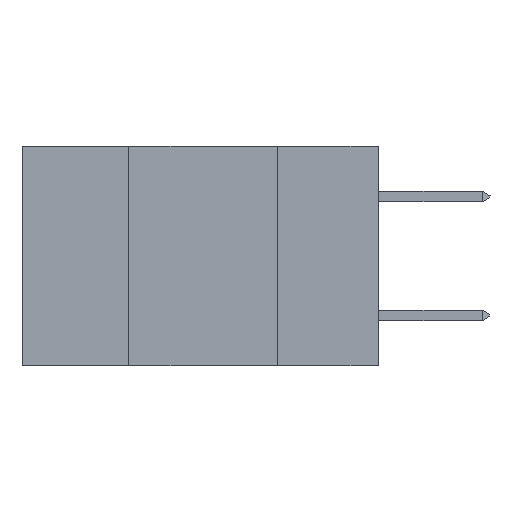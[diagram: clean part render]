
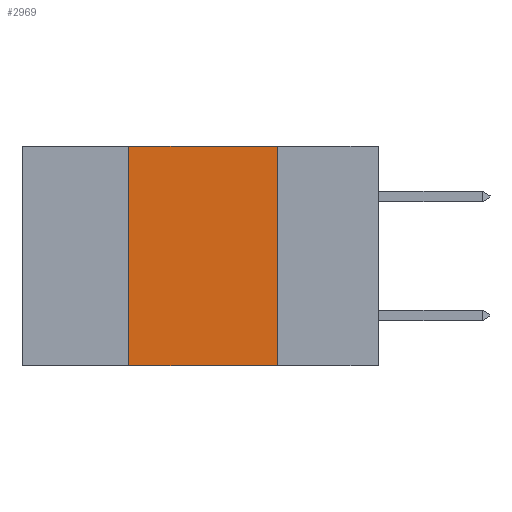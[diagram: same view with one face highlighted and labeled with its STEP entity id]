
A CAD part, left-side view. The second image highlights one B-rep face of the part: STEP entity #2969.
In plain terms, the highlighted planar face has unit normal (-1, 0, 0).
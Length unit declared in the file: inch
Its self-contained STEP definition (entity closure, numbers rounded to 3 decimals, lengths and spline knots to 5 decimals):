
#206 = AXIS2_PLACEMENT_3D ( 'NONE', #6685, #3873, #6590 ) ;
#290 = CARTESIAN_POINT ( 'NONE',  ( 0., 0.42, -0.37 ) ) ;
#675 = VECTOR ( 'NONE', #8273, 39.37008 ) ;
#930 = DIRECTION ( 'NONE',  ( 0., 0., -1. ) ) ;
#960 = VERTEX_POINT ( 'NONE', #290 ) ;
#1196 = PLANE ( 'NONE',  #206 ) ;
#1457 = LINE ( 'NONE', #4963, #675 ) ;
#1615 = CARTESIAN_POINT ( 'NONE',  ( 0., 0.17, 0. ) ) ;
#1866 = LINE ( 'NONE', #7361, #2971 ) ;
#1905 = EDGE_CURVE ( 'NONE', #960, #2613, #1866, .T. ) ;
#1963 = FACE_OUTER_BOUND ( 'NONE', #2246, .T. ) ;
#2007 = ORIENTED_EDGE ( 'NONE', *, *, #1905, .T. ) ;
#2048 = EDGE_CURVE ( 'NONE', #960, #8710, #7656, .T. ) ;
#2240 = ORIENTED_EDGE ( 'NONE', *, *, #2048, .F. ) ;
#2246 = EDGE_LOOP ( 'NONE', ( #3797, #7391, #2240, #2007 ) ) ;
#2274 = LINE ( 'NONE', #7089, #4988 ) ;
#2612 = DIRECTION ( 'NONE',  ( 0., -1., 0. ) ) ;
#2613 = VERTEX_POINT ( 'NONE', #2953 ) ;
#2637 = VERTEX_POINT ( 'NONE', #1615 ) ;
#2910 = DIRECTION ( 'NONE',  ( 0., 0., 1. ) ) ;
#2953 = CARTESIAN_POINT ( 'NONE',  ( 0., 0.17, -0.37 ) ) ;
#2969 = ADVANCED_FACE ( 'NONE', ( #1963 ), #1196, .F. ) ;
#2971 = VECTOR ( 'NONE', #2612, 39.37008 ) ;
#3797 = ORIENTED_EDGE ( 'NONE', *, *, #3976, .F. ) ;
#3873 = DIRECTION ( 'NONE',  ( 1., 0., 0. ) ) ;
#3976 = EDGE_CURVE ( 'NONE', #2637, #2613, #2274, .T. ) ;
#4720 = CARTESIAN_POINT ( 'NONE',  ( 0., 0.42, 0. ) ) ;
#4963 = CARTESIAN_POINT ( 'NONE',  ( 0., 0.6, 0. ) ) ;
#4988 = VECTOR ( 'NONE', #930, 39.37008 ) ;
#5397 = EDGE_CURVE ( 'NONE', #8710, #2637, #1457, .T. ) ;
#5407 = CARTESIAN_POINT ( 'NONE',  ( 0., 0.42, -0.37 ) ) ;
#6590 = DIRECTION ( 'NONE',  ( 0., 0., -1. ) ) ;
#6685 = CARTESIAN_POINT ( 'NONE',  ( 0., 0.6, 0. ) ) ;
#7089 = CARTESIAN_POINT ( 'NONE',  ( 0., 0.17, -0.37 ) ) ;
#7329 = VECTOR ( 'NONE', #2910, 39.37008 ) ;
#7361 = CARTESIAN_POINT ( 'NONE',  ( 0., 0.6, -0.37 ) ) ;
#7391 = ORIENTED_EDGE ( 'NONE', *, *, #5397, .F. ) ;
#7656 = LINE ( 'NONE', #5407, #7329 ) ;
#8273 = DIRECTION ( 'NONE',  ( 0., -1., 0. ) ) ;
#8710 = VERTEX_POINT ( 'NONE', #4720 ) ;
